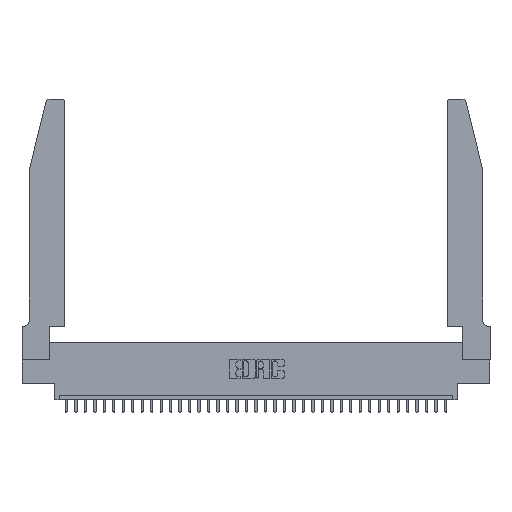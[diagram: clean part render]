
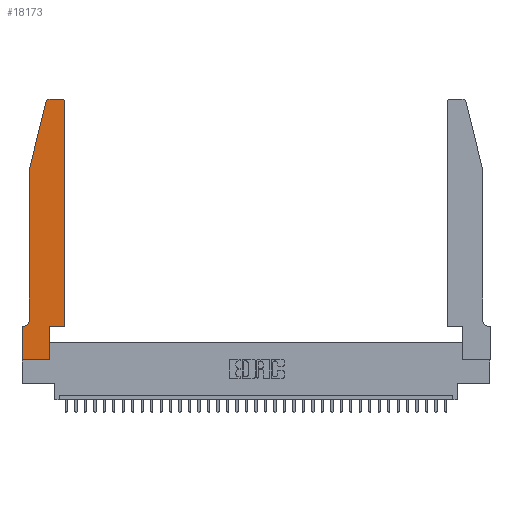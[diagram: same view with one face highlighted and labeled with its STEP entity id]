
A CAD part, top view. The second image highlights one B-rep face of the part: STEP entity #18173.
In plain terms, the highlighted planar face has unit normal (0, 0, 1).
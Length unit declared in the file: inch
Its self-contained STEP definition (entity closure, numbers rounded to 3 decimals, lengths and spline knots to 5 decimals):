
#5 = LINE ( 'NONE', #12408, #21283 ) ;
#321 = VERTEX_POINT ( 'NONE', #11260 ) ;
#646 = EDGE_CURVE ( 'NONE', #17591, #17416, #14484, .T. ) ;
#906 = DIRECTION ( 'NONE',  ( -1., 0., 0. ) ) ;
#1779 = DIRECTION ( 'NONE',  ( -1., 0., 0. ) ) ;
#2055 = ORIENTED_EDGE ( 'NONE', *, *, #10328, .T. ) ;
#2083 = EDGE_CURVE ( 'NONE', #18308, #20587, #3832, .T. ) ;
#2624 = ORIENTED_EDGE ( 'NONE', *, *, #30559, .T. ) ;
#2996 = VERTEX_POINT ( 'NONE', #31895 ) ;
#3392 = CARTESIAN_POINT ( 'NONE',  ( 0.4505, 2.72, 0.37 ) ) ;
#3832 = LINE ( 'NONE', #25418, #11616 ) ;
#4216 = ORIENTED_EDGE ( 'NONE', *, *, #8780, .T. ) ;
#4309 = VERTEX_POINT ( 'NONE', #14984 ) ;
#4552 = EDGE_CURVE ( 'NONE', #31355, #4309, #9297, .T. ) ;
#4636 = ORIENTED_EDGE ( 'NONE', *, *, #29243, .T. ) ;
#4651 = AXIS2_PLACEMENT_3D ( 'NONE', #11079, #5484, #27967 ) ;
#4883 = CARTESIAN_POINT ( 'NONE',  ( 0., 0.35, 0.37 ) ) ;
#5461 = CIRCLE ( 'NONE', #9541, 0.03 ) ;
#5484 = DIRECTION ( 'NONE',  ( 0., 0., 1. ) ) ;
#5846 = DIRECTION ( 'NONE',  ( 1., 0., 0. ) ) ;
#6102 = ORIENTED_EDGE ( 'NONE', *, *, #4552, .T. ) ;
#6200 = FACE_OUTER_BOUND ( 'NONE', #11627, .T. ) ;
#6465 = DIRECTION ( 'NONE',  ( 0., 0., 1. ) ) ;
#6817 = ORIENTED_EDGE ( 'NONE', *, *, #646, .T. ) ;
#6917 = DIRECTION ( 'NONE',  ( 0., 0., 1. ) ) ;
#6962 = DIRECTION ( 'NONE',  ( 0., -1., 0. ) ) ;
#7015 = VERTEX_POINT ( 'NONE', #9078 ) ;
#7201 = LINE ( 'NONE', #20793, #28457 ) ;
#8276 = AXIS2_PLACEMENT_3D ( 'NONE', #28714, #6465, #9150 ) ;
#8550 = VECTOR ( 'NONE', #33673, 39.37008 ) ;
#8780 = EDGE_CURVE ( 'NONE', #28820, #18308, #7201, .T. ) ;
#8883 = CARTESIAN_POINT ( 'NONE',  ( 0.25487, 2.72718, 0.37 ) ) ;
#9078 = CARTESIAN_POINT ( 'NONE',  ( 0.0755, 2., 0.37 ) ) ;
#9150 = DIRECTION ( 'NONE',  ( 1., 0., 0. ) ) ;
#9297 = LINE ( 'NONE', #31729, #30586 ) ;
#9514 = DIRECTION ( 'NONE',  ( 0., 1., 0. ) ) ;
#9541 = AXIS2_PLACEMENT_3D ( 'NONE', #28766, #6917, #20378 ) ;
#9671 = ORIENTED_EDGE ( 'NONE', *, *, #15312, .T. ) ;
#10328 = EDGE_CURVE ( 'NONE', #20727, #7015, #16155, .T. ) ;
#10903 = ORIENTED_EDGE ( 'NONE', *, *, #2083, .T. ) ;
#11079 = CARTESIAN_POINT ( 'NONE',  ( 0., 0.35, 0.37 ) ) ;
#11140 = CARTESIAN_POINT ( 'NONE',  ( 0.0755, 2., 0.37 ) ) ;
#11260 = CARTESIAN_POINT ( 'NONE',  ( 0.0755, 0.42, 0.37 ) ) ;
#11264 = CARTESIAN_POINT ( 'NONE',  ( 0.2865, 0.35, 0.37 ) ) ;
#11616 = VECTOR ( 'NONE', #5846, 39.37008 ) ;
#11627 = EDGE_LOOP ( 'NONE', ( #6817, #32132, #2055, #23995, #27211, #2624, #4216, #10903, #9671, #6102, #28891, #4636 ) ) ;
#12408 = CARTESIAN_POINT ( 'NONE',  ( 0.0755, 0.35, 0.37 ) ) ;
#13295 = CARTESIAN_POINT ( 'NONE',  ( 0.4505, 0.35, 0.37 ) ) ;
#14484 = LINE ( 'NONE', #18057, #30996 ) ;
#14725 = DIRECTION ( 'NONE',  ( 0., 0., -1. ) ) ;
#14984 = CARTESIAN_POINT ( 'NONE',  ( 0.4505, 0.35, 0.37 ) ) ;
#15312 = EDGE_CURVE ( 'NONE', #20587, #31355, #27317, .T. ) ;
#15986 = AXIS2_PLACEMENT_3D ( 'NONE', #20178, #14725, #906 ) ;
#16155 = LINE ( 'NONE', #29131, #34809 ) ;
#16985 = DIRECTION ( 'NONE',  ( 0., 1., 0. ) ) ;
#16996 = VECTOR ( 'NONE', #16985, 39.37008 ) ;
#17416 = VERTEX_POINT ( 'NONE', #29406 ) ;
#17476 = CARTESIAN_POINT ( 'NONE',  ( 0., 0., 0.37 ) ) ;
#17591 = VERTEX_POINT ( 'NONE', #28699 ) ;
#17677 = CIRCLE ( 'NONE', #8276, 0.03 ) ;
#18057 = CARTESIAN_POINT ( 'NONE',  ( 0.2605, 2.75, 0.37 ) ) ;
#18173 = ADVANCED_FACE ( 'NONE', ( #6200 ), #35824, .T. ) ;
#18308 = VERTEX_POINT ( 'NONE', #17476 ) ;
#18481 = CIRCLE ( 'NONE', #15986, 0.07 ) ;
#18919 = EDGE_CURVE ( 'NONE', #4309, #25011, #24452, .T. ) ;
#18936 = CARTESIAN_POINT ( 'NONE',  ( 0.2865, 0.35, 0.37 ) ) ;
#19347 = DIRECTION ( 'NONE',  ( 1., 0., 0. ) ) ;
#20178 = CARTESIAN_POINT ( 'NONE',  ( 0.0055, 0.42, 0.37 ) ) ;
#20378 = DIRECTION ( 'NONE',  ( 1., 0., 0. ) ) ;
#20587 = VERTEX_POINT ( 'NONE', #27238 ) ;
#20727 = VERTEX_POINT ( 'NONE', #8883 ) ;
#20793 = CARTESIAN_POINT ( 'NONE',  ( 0., 0., 0.37 ) ) ;
#21283 = VECTOR ( 'NONE', #1779, 39.37008 ) ;
#22175 = EDGE_CURVE ( 'NONE', #7015, #321, #31575, .T. ) ;
#22957 = EDGE_CURVE ( 'NONE', #17416, #20727, #17677, .T. ) ;
#23995 = ORIENTED_EDGE ( 'NONE', *, *, #22175, .T. ) ;
#24046 = EDGE_CURVE ( 'NONE', #321, #2996, #18481, .T. ) ;
#24452 = LINE ( 'NONE', #13295, #16996 ) ;
#25011 = VERTEX_POINT ( 'NONE', #3392 ) ;
#25418 = CARTESIAN_POINT ( 'NONE',  ( 0., 0., 0.37 ) ) ;
#26430 = VECTOR ( 'NONE', #9514, 39.37008 ) ;
#27211 = ORIENTED_EDGE ( 'NONE', *, *, #24046, .T. ) ;
#27238 = CARTESIAN_POINT ( 'NONE',  ( 0.2865, 0., 0.37 ) ) ;
#27317 = LINE ( 'NONE', #11264, #26430 ) ;
#27967 = DIRECTION ( 'NONE',  ( 1., 0., 0. ) ) ;
#28457 = VECTOR ( 'NONE', #6962, 39.37008 ) ;
#28699 = CARTESIAN_POINT ( 'NONE',  ( 0.4205, 2.75, 0.37 ) ) ;
#28714 = CARTESIAN_POINT ( 'NONE',  ( 0.284, 2.72, 0.37 ) ) ;
#28766 = CARTESIAN_POINT ( 'NONE',  ( 0.4205, 2.72, 0.37 ) ) ;
#28820 = VERTEX_POINT ( 'NONE', #4883 ) ;
#28891 = ORIENTED_EDGE ( 'NONE', *, *, #18919, .T. ) ;
#29131 = CARTESIAN_POINT ( 'NONE',  ( 0.0755, 2., 0.37 ) ) ;
#29243 = EDGE_CURVE ( 'NONE', #25011, #17591, #5461, .T. ) ;
#29364 = DIRECTION ( 'NONE',  ( -0.239, -0.971, 0. ) ) ;
#29406 = CARTESIAN_POINT ( 'NONE',  ( 0.284, 2.75, 0.37 ) ) ;
#30547 = DIRECTION ( 'NONE',  ( -1., 0., 0. ) ) ;
#30559 = EDGE_CURVE ( 'NONE', #2996, #28820, #5, .T. ) ;
#30586 = VECTOR ( 'NONE', #19347, 39.37008 ) ;
#30996 = VECTOR ( 'NONE', #30547, 39.37008 ) ;
#31355 = VERTEX_POINT ( 'NONE', #18936 ) ;
#31575 = LINE ( 'NONE', #11140, #8550 ) ;
#31729 = CARTESIAN_POINT ( 'NONE',  ( 0.4505, 0.35, 0.37 ) ) ;
#31895 = CARTESIAN_POINT ( 'NONE',  ( 0.0055, 0.35, 0.37 ) ) ;
#32132 = ORIENTED_EDGE ( 'NONE', *, *, #22957, .T. ) ;
#33673 = DIRECTION ( 'NONE',  ( 0., -1., 0. ) ) ;
#34809 = VECTOR ( 'NONE', #29364, 39.37008 ) ;
#35824 = PLANE ( 'NONE',  #4651 ) ;
